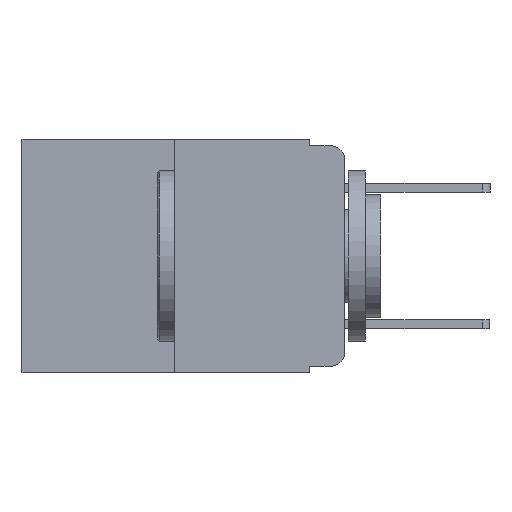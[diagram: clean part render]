
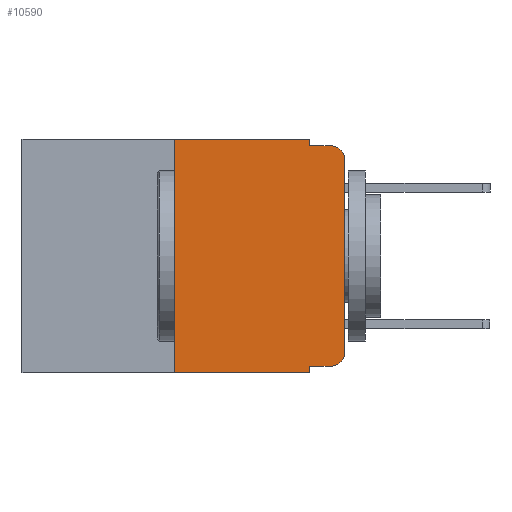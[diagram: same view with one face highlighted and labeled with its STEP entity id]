
A CAD part, left-side view. The second image highlights one B-rep face of the part: STEP entity #10590.
In plain terms, the highlighted planar face has unit normal (-1, 0, 0).
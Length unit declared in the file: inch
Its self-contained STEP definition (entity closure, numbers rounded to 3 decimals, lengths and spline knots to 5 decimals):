
#132 = DIRECTION ( 'NONE',  ( 1., 0., 0. ) ) ;
#268 = VERTEX_POINT ( 'NONE', #1921 ) ;
#393 = ORIENTED_EDGE ( 'NONE', *, *, #8284, .T. ) ;
#412 = VERTEX_POINT ( 'NONE', #6453 ) ;
#675 = VECTOR ( 'NONE', #3663, 39.37008 ) ;
#866 = VERTEX_POINT ( 'NONE', #883 ) ;
#883 = CARTESIAN_POINT ( 'NONE',  ( 0., 0.02, -0.01 ) ) ;
#1039 = CARTESIAN_POINT ( 'NONE',  ( 0., 0.051, 0. ) ) ;
#1130 = CARTESIAN_POINT ( 'NONE',  ( 0., 0.473, -0.343 ) ) ;
#1197 = CARTESIAN_POINT ( 'NONE',  ( 0., 0.02, -0.03 ) ) ;
#1241 = CARTESIAN_POINT ( 'NONE',  ( 0., 0., -0.313 ) ) ;
#1406 = DIRECTION ( 'NONE',  ( 0., 0., -1. ) ) ;
#1408 = ORIENTED_EDGE ( 'NONE', *, *, #7154, .F. ) ;
#1422 = VECTOR ( 'NONE', #3943, 39.37008 ) ;
#1439 = ORIENTED_EDGE ( 'NONE', *, *, #5363, .F. ) ;
#1721 = CARTESIAN_POINT ( 'NONE',  ( 0., 0.25, 0. ) ) ;
#1860 = CARTESIAN_POINT ( 'NONE',  ( 0., 0.051, -0.01 ) ) ;
#1921 = CARTESIAN_POINT ( 'NONE',  ( 0., 0.051, -0.333 ) ) ;
#1926 = LINE ( 'NONE', #3089, #2252 ) ;
#1995 = AXIS2_PLACEMENT_3D ( 'NONE', #7703, #3883, #3865 ) ;
#2074 = LINE ( 'NONE', #11634, #6830 ) ;
#2245 = DIRECTION ( 'NONE',  ( 0., 0., -1. ) ) ;
#2252 = VECTOR ( 'NONE', #9329, 39.37008 ) ;
#2270 = VERTEX_POINT ( 'NONE', #6478 ) ;
#2430 = ORIENTED_EDGE ( 'NONE', *, *, #4740, .T. ) ;
#2466 = CARTESIAN_POINT ( 'NONE',  ( 0., 0., -0.03 ) ) ;
#2698 = EDGE_CURVE ( 'NONE', #9127, #11981, #4420, .T. ) ;
#2862 = ORIENTED_EDGE ( 'NONE', *, *, #4989, .F. ) ;
#3089 = CARTESIAN_POINT ( 'NONE',  ( 0., 0., 0. ) ) ;
#3425 = LINE ( 'NONE', #9662, #675 ) ;
#3453 = EDGE_CURVE ( 'NONE', #8143, #5511, #10450, .T. ) ;
#3663 = DIRECTION ( 'NONE',  ( 0., 0., 1. ) ) ;
#3865 = DIRECTION ( 'NONE',  ( 0., 0., -1. ) ) ;
#3883 = DIRECTION ( 'NONE',  ( -1., 0., 0. ) ) ;
#3890 = ORIENTED_EDGE ( 'NONE', *, *, #2698, .T. ) ;
#3940 = VECTOR ( 'NONE', #1406, 39.37008 ) ;
#3943 = DIRECTION ( 'NONE',  ( 0., -1., 0. ) ) ;
#4420 = LINE ( 'NONE', #1130, #1422 ) ;
#4477 = CARTESIAN_POINT ( 'NONE',  ( 0., 0.473, 0. ) ) ;
#4740 = EDGE_CURVE ( 'NONE', #268, #8143, #2074, .T. ) ;
#4984 = ORIENTED_EDGE ( 'NONE', *, *, #8843, .T. ) ;
#4989 = EDGE_CURVE ( 'NONE', #7877, #2270, #11902, .T. ) ;
#5038 = CARTESIAN_POINT ( 'NONE',  ( 0., 0.02, -0.333 ) ) ;
#5087 = DIRECTION ( 'NONE',  ( 0., 0., -1. ) ) ;
#5340 = LINE ( 'NONE', #10251, #11964 ) ;
#5363 = EDGE_CURVE ( 'NONE', #268, #11981, #10955, .T. ) ;
#5414 = CARTESIAN_POINT ( 'NONE',  ( 0., 0.25, -0.343 ) ) ;
#5511 = VERTEX_POINT ( 'NONE', #1241 ) ;
#5833 = ORIENTED_EDGE ( 'NONE', *, *, #7707, .F. ) ;
#6022 = ORIENTED_EDGE ( 'NONE', *, *, #3453, .T. ) ;
#6453 = CARTESIAN_POINT ( 'NONE',  ( 0., 0.051, -0.01 ) ) ;
#6478 = CARTESIAN_POINT ( 'NONE',  ( 0., 0.051, 0. ) ) ;
#6534 = CARTESIAN_POINT ( 'NONE',  ( 0., 0.051, -0.343 ) ) ;
#6563 = EDGE_CURVE ( 'NONE', #9127, #7877, #3425, .T. ) ;
#6674 = ORIENTED_EDGE ( 'NONE', *, *, #6563, .F. ) ;
#6830 = VECTOR ( 'NONE', #9403, 39.37008 ) ;
#7017 = DIRECTION ( 'NONE',  ( 0., 0., -1. ) ) ;
#7154 = EDGE_CURVE ( 'NONE', #2270, #412, #5340, .T. ) ;
#7489 = DIRECTION ( 'NONE',  ( 0., -1., 0. ) ) ;
#7703 = CARTESIAN_POINT ( 'NONE',  ( 0., 0.02, -0.313 ) ) ;
#7707 = EDGE_CURVE ( 'NONE', #412, #866, #11413, .T. ) ;
#7799 = DIRECTION ( 'NONE',  ( -1., 0., 0. ) ) ;
#7876 = VERTEX_POINT ( 'NONE', #2466 ) ;
#7877 = VERTEX_POINT ( 'NONE', #1721 ) ;
#8097 = AXIS2_PLACEMENT_3D ( 'NONE', #10386, #132, #7017 ) ;
#8143 = VERTEX_POINT ( 'NONE', #5038 ) ;
#8284 = EDGE_CURVE ( 'NONE', #7876, #866, #10012, .T. ) ;
#8843 = EDGE_CURVE ( 'NONE', #5511, #7876, #1926, .T. ) ;
#8851 = VECTOR ( 'NONE', #7489, 39.37008 ) ;
#9127 = VERTEX_POINT ( 'NONE', #5414 ) ;
#9329 = DIRECTION ( 'NONE',  ( 0., 0., 1. ) ) ;
#9403 = DIRECTION ( 'NONE',  ( 0., -1., 0. ) ) ;
#9419 = AXIS2_PLACEMENT_3D ( 'NONE', #1197, #7799, #2245 ) ;
#9583 = VECTOR ( 'NONE', #10680, 39.37008 ) ;
#9662 = CARTESIAN_POINT ( 'NONE',  ( 0., 0.25, 0. ) ) ;
#10012 = CIRCLE ( 'NONE', #9419, 0.02 ) ;
#10251 = CARTESIAN_POINT ( 'NONE',  ( 0., 0.051, 0. ) ) ;
#10347 = PLANE ( 'NONE',  #8097 ) ;
#10386 = CARTESIAN_POINT ( 'NONE',  ( 0., 0.473, 0. ) ) ;
#10450 = CIRCLE ( 'NONE', #1995, 0.02 ) ;
#10590 = ADVANCED_FACE ( 'NONE', ( #11196 ), #10347, .F. ) ;
#10680 = DIRECTION ( 'NONE',  ( 0., -1., 0. ) ) ;
#10955 = LINE ( 'NONE', #1039, #3940 ) ;
#11196 = FACE_OUTER_BOUND ( 'NONE', #11909, .T. ) ;
#11413 = LINE ( 'NONE', #1860, #8851 ) ;
#11634 = CARTESIAN_POINT ( 'NONE',  ( 0., 0.051, -0.333 ) ) ;
#11902 = LINE ( 'NONE', #4477, #9583 ) ;
#11909 = EDGE_LOOP ( 'NONE', ( #4984, #393, #5833, #1408, #2862, #6674, #3890, #1439, #2430, #6022 ) ) ;
#11964 = VECTOR ( 'NONE', #5087, 39.37008 ) ;
#11981 = VERTEX_POINT ( 'NONE', #6534 ) ;
